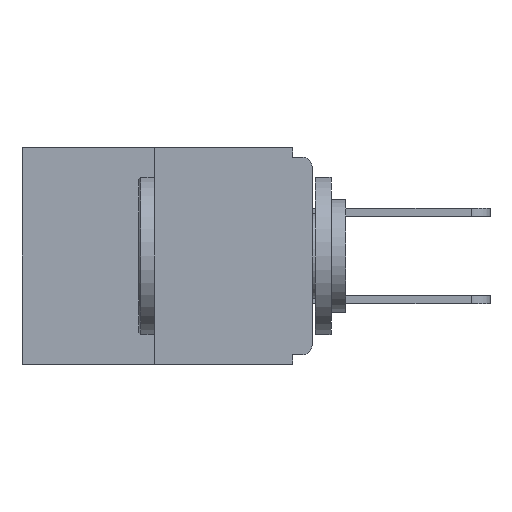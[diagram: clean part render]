
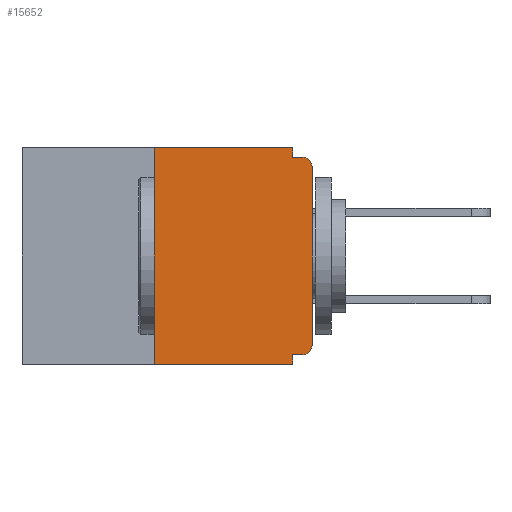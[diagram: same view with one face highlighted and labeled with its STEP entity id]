
A CAD part, left-side view. The second image highlights one B-rep face of the part: STEP entity #15652.
In plain terms, the highlighted planar face has unit normal (-1, 0, 0).
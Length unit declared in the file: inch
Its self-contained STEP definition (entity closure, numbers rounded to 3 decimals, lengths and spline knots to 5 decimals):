
#992 = DIRECTION ( 'NONE',  ( -1., 0., 0. ) ) ;
#1359 = VERTEX_POINT ( 'NONE', #11609 ) ;
#1587 = CARTESIAN_POINT ( 'NONE',  ( 0., 0., -0.313 ) ) ;
#1704 = LINE ( 'NONE', #5470, #12163 ) ;
#2238 = CARTESIAN_POINT ( 'NONE',  ( 0., 0.031, 0. ) ) ;
#2512 = CARTESIAN_POINT ( 'NONE',  ( 0., 0.25, 0. ) ) ;
#2576 = DIRECTION ( 'NONE',  ( 0., 0., -1. ) ) ;
#2705 = VERTEX_POINT ( 'NONE', #16751 ) ;
#3398 = EDGE_CURVE ( 'NONE', #21399, #2705, #6950, .T. ) ;
#3673 = EDGE_CURVE ( 'NONE', #21934, #2705, #10326, .T. ) ;
#4078 = DIRECTION ( 'NONE',  ( 0., 1., 0. ) ) ;
#4270 = VERTEX_POINT ( 'NONE', #19833 ) ;
#4358 = ORIENTED_EDGE ( 'NONE', *, *, #8790, .F. ) ;
#4873 = DIRECTION ( 'NONE',  ( 0., 0., -1. ) ) ;
#5086 = CARTESIAN_POINT ( 'NONE',  ( 0., 0.031, 0. ) ) ;
#5254 = CARTESIAN_POINT ( 'NONE',  ( 0., 0.015, -0.328 ) ) ;
#5289 = VERTEX_POINT ( 'NONE', #15899 ) ;
#5380 = PLANE ( 'NONE',  #15879 ) ;
#5400 = ORIENTED_EDGE ( 'NONE', *, *, #9306, .F. ) ;
#5470 = CARTESIAN_POINT ( 'NONE',  ( 0., 0.46, -0.343 ) ) ;
#5763 = VERTEX_POINT ( 'NONE', #5254 ) ;
#5868 = CARTESIAN_POINT ( 'NONE',  ( 0., 0., -0.03 ) ) ;
#6109 = CARTESIAN_POINT ( 'NONE',  ( 0., 0.46, 0. ) ) ;
#6176 = ORIENTED_EDGE ( 'NONE', *, *, #15988, .F. ) ;
#6829 = DIRECTION ( 'NONE',  ( 0., 0., -1. ) ) ;
#6856 = EDGE_CURVE ( 'NONE', #11672, #21399, #21412, .T. ) ;
#6950 = CIRCLE ( 'NONE', #22598, 0.015 ) ;
#7003 = DIRECTION ( 'NONE',  ( 0., -1., 0. ) ) ;
#7125 = CARTESIAN_POINT ( 'NONE',  ( 0., 0.46, 0. ) ) ;
#8790 = EDGE_CURVE ( 'NONE', #1359, #10277, #15680, .T. ) ;
#9306 = EDGE_CURVE ( 'NONE', #5763, #1359, #17334, .T. ) ;
#9858 = CARTESIAN_POINT ( 'NONE',  ( 0., 0.015, -0.03 ) ) ;
#10172 = DIRECTION ( 'NONE',  ( 0., 0., 1. ) ) ;
#10277 = VERTEX_POINT ( 'NONE', #18346 ) ;
#10326 = LINE ( 'NONE', #14095, #17674 ) ;
#10429 = VECTOR ( 'NONE', #6829, 39.37008 ) ;
#10647 = DIRECTION ( 'NONE',  ( 0., 0., -1. ) ) ;
#11591 = EDGE_CURVE ( 'NONE', #16278, #21934, #23493, .T. ) ;
#11609 = CARTESIAN_POINT ( 'NONE',  ( 0., 0.031, -0.328 ) ) ;
#11672 = VERTEX_POINT ( 'NONE', #1587 ) ;
#12163 = VECTOR ( 'NONE', #21623, 39.37008 ) ;
#12388 = VECTOR ( 'NONE', #18765, 39.37008 ) ;
#12636 = DIRECTION ( 'NONE',  ( 1., 0., 0. ) ) ;
#12992 = ORIENTED_EDGE ( 'NONE', *, *, #18256, .T. ) ;
#13131 = EDGE_CURVE ( 'NONE', #4270, #16278, #19751, .T. ) ;
#14095 = CARTESIAN_POINT ( 'NONE',  ( 0., 0., -0.015 ) ) ;
#14258 = LINE ( 'NONE', #2512, #22816 ) ;
#14457 = EDGE_CURVE ( 'NONE', #5763, #11672, #17145, .T. ) ;
#15104 = ORIENTED_EDGE ( 'NONE', *, *, #6856, .T. ) ;
#15214 = CARTESIAN_POINT ( 'NONE',  ( 0., 0.015, -0.313 ) ) ;
#15226 = CARTESIAN_POINT ( 'NONE',  ( 0., 0., 0. ) ) ;
#15373 = VECTOR ( 'NONE', #10647, 39.37008 ) ;
#15652 = ADVANCED_FACE ( 'NONE', ( #18250 ), #5380, .F. ) ;
#15680 = LINE ( 'NONE', #19594, #15373 ) ;
#15879 = AXIS2_PLACEMENT_3D ( 'NONE', #7125, #12636, #19767 ) ;
#15899 = CARTESIAN_POINT ( 'NONE',  ( 0., 0.25, -0.343 ) ) ;
#15988 = EDGE_CURVE ( 'NONE', #5289, #4270, #14258, .T. ) ;
#16019 = AXIS2_PLACEMENT_3D ( 'NONE', #15214, #992, #4873 ) ;
#16106 = CARTESIAN_POINT ( 'NONE',  ( 0., 0.031, -0.015 ) ) ;
#16207 = VECTOR ( 'NONE', #4078, 39.37008 ) ;
#16278 = VERTEX_POINT ( 'NONE', #2238 ) ;
#16568 = VECTOR ( 'NONE', #10172, 39.37008 ) ;
#16751 = CARTESIAN_POINT ( 'NONE',  ( 0., 0.015, -0.015 ) ) ;
#17047 = ORIENTED_EDGE ( 'NONE', *, *, #11591, .F. ) ;
#17073 = CARTESIAN_POINT ( 'NONE',  ( 0., 0., -0.328 ) ) ;
#17145 = CIRCLE ( 'NONE', #16019, 0.015 ) ;
#17151 = ORIENTED_EDGE ( 'NONE', *, *, #3398, .T. ) ;
#17334 = LINE ( 'NONE', #17073, #16207 ) ;
#17674 = VECTOR ( 'NONE', #7003, 39.37008 ) ;
#18250 = FACE_OUTER_BOUND ( 'NONE', #20826, .T. ) ;
#18256 = EDGE_CURVE ( 'NONE', #5289, #10277, #1704, .T. ) ;
#18346 = CARTESIAN_POINT ( 'NONE',  ( 0., 0.031, -0.343 ) ) ;
#18765 = DIRECTION ( 'NONE',  ( 0., -1., 0. ) ) ;
#19594 = CARTESIAN_POINT ( 'NONE',  ( 0., 0.031, -0.343 ) ) ;
#19751 = LINE ( 'NONE', #6109, #12388 ) ;
#19767 = DIRECTION ( 'NONE',  ( 0., 0., -1. ) ) ;
#19833 = CARTESIAN_POINT ( 'NONE',  ( 0., 0.25, 0. ) ) ;
#20645 = DIRECTION ( 'NONE',  ( 0., 0., 1. ) ) ;
#20698 = ORIENTED_EDGE ( 'NONE', *, *, #13131, .F. ) ;
#20808 = ORIENTED_EDGE ( 'NONE', *, *, #3673, .F. ) ;
#20826 = EDGE_LOOP ( 'NONE', ( #20698, #6176, #12992, #4358, #5400, #21675, #15104, #17151, #20808, #17047 ) ) ;
#21399 = VERTEX_POINT ( 'NONE', #5868 ) ;
#21412 = LINE ( 'NONE', #15226, #16568 ) ;
#21623 = DIRECTION ( 'NONE',  ( 0., -1., 0. ) ) ;
#21675 = ORIENTED_EDGE ( 'NONE', *, *, #14457, .T. ) ;
#21934 = VERTEX_POINT ( 'NONE', #16106 ) ;
#22539 = DIRECTION ( 'NONE',  ( -1., 0., 0. ) ) ;
#22598 = AXIS2_PLACEMENT_3D ( 'NONE', #9858, #22539, #2576 ) ;
#22816 = VECTOR ( 'NONE', #20645, 39.37008 ) ;
#23493 = LINE ( 'NONE', #5086, #10429 ) ;
